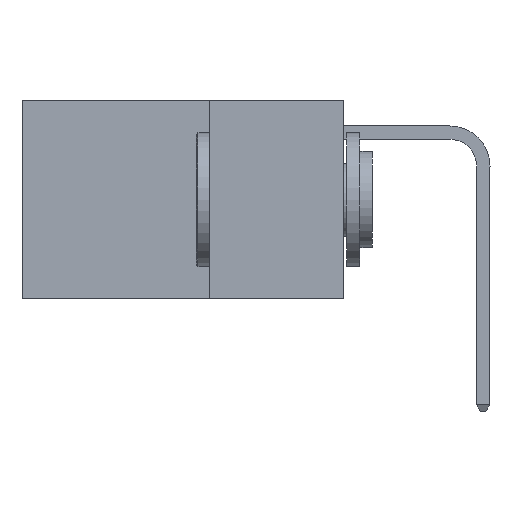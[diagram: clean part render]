
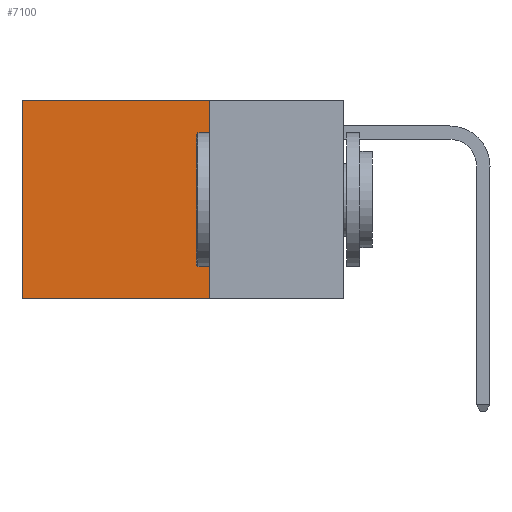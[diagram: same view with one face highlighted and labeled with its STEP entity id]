
A CAD part, left-side view. The second image highlights one B-rep face of the part: STEP entity #7100.
In plain terms, the highlighted planar face has unit normal (-1, 0, 0).
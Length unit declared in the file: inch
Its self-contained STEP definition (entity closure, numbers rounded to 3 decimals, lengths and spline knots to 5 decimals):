
#24 = DIRECTION ( 'NONE',  ( 0., 0., -1. ) ) ;
#1250 = DIRECTION ( 'NONE',  ( 0., 1., 0. ) ) ;
#1279 = FACE_OUTER_BOUND ( 'NONE', #3104, .T. ) ;
#2738 = LINE ( 'NONE', #14993, #12635 ) ;
#2809 = LINE ( 'NONE', #4425, #5746 ) ;
#3104 = EDGE_LOOP ( 'NONE', ( #8644, #9601, #10621, #10401 ) ) ;
#4425 = CARTESIAN_POINT ( 'NONE',  ( 0.2625, 0.6, 0. ) ) ;
#4515 = VECTOR ( 'NONE', #1250, 39.37008 ) ;
#4908 = VERTEX_POINT ( 'NONE', #10575 ) ;
#5746 = VECTOR ( 'NONE', #15501, 39.37008 ) ;
#5965 = EDGE_CURVE ( 'NONE', #16295, #12050, #2809, .T. ) ;
#6110 = CARTESIAN_POINT ( 'NONE',  ( 0.2625, 0.6, 0. ) ) ;
#6923 = AXIS2_PLACEMENT_3D ( 'NONE', #18064, #8706, #24 ) ;
#7100 = ADVANCED_FACE ( 'NONE', ( #1279 ), #16826, .F. ) ;
#7656 = VERTEX_POINT ( 'NONE', #9725 ) ;
#8255 = DIRECTION ( 'NONE',  ( 0., 0., -1. ) ) ;
#8378 = EDGE_CURVE ( 'NONE', #4908, #7656, #2738, .T. ) ;
#8644 = ORIENTED_EDGE ( 'NONE', *, *, #5965, .T. ) ;
#8706 = DIRECTION ( 'NONE',  ( 1., 0., 0. ) ) ;
#9390 = CARTESIAN_POINT ( 'NONE',  ( 0.2625, 0.6, -0.37 ) ) ;
#9601 = ORIENTED_EDGE ( 'NONE', *, *, #16735, .F. ) ;
#9725 = CARTESIAN_POINT ( 'NONE',  ( 0.2625, 0.25, -0.37 ) ) ;
#9989 = LINE ( 'NONE', #16046, #16732 ) ;
#10401 = ORIENTED_EDGE ( 'NONE', *, *, #11298, .T. ) ;
#10575 = CARTESIAN_POINT ( 'NONE',  ( 0.2625, 0.25, 0. ) ) ;
#10621 = ORIENTED_EDGE ( 'NONE', *, *, #8378, .F. ) ;
#11298 = EDGE_CURVE ( 'NONE', #4908, #16295, #9989, .T. ) ;
#12050 = VERTEX_POINT ( 'NONE', #9390 ) ;
#12635 = VECTOR ( 'NONE', #8255, 39.37008 ) ;
#14993 = CARTESIAN_POINT ( 'NONE',  ( 0.2625, 0.25, 0. ) ) ;
#15501 = DIRECTION ( 'NONE',  ( 0., 0., -1. ) ) ;
#15559 = LINE ( 'NONE', #17851, #4515 ) ;
#16046 = CARTESIAN_POINT ( 'NONE',  ( 0.2625, 0.25, 0. ) ) ;
#16295 = VERTEX_POINT ( 'NONE', #6110 ) ;
#16732 = VECTOR ( 'NONE', #17347, 39.37008 ) ;
#16735 = EDGE_CURVE ( 'NONE', #7656, #12050, #15559, .T. ) ;
#16826 = PLANE ( 'NONE',  #6923 ) ;
#17347 = DIRECTION ( 'NONE',  ( 0., 1., 0. ) ) ;
#17851 = CARTESIAN_POINT ( 'NONE',  ( 0.2625, 0.25, -0.37 ) ) ;
#18064 = CARTESIAN_POINT ( 'NONE',  ( 0.2625, 0.25, 0. ) ) ;
